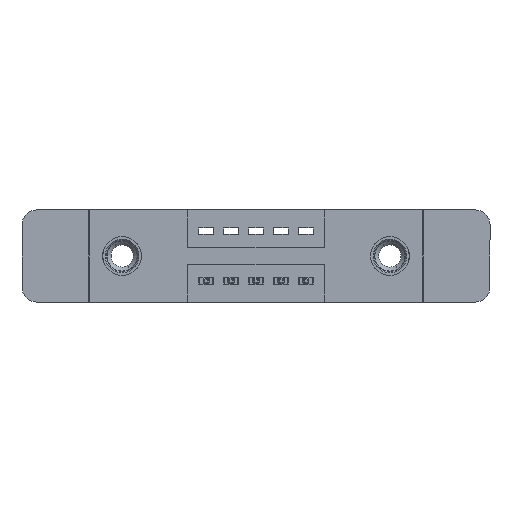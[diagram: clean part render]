
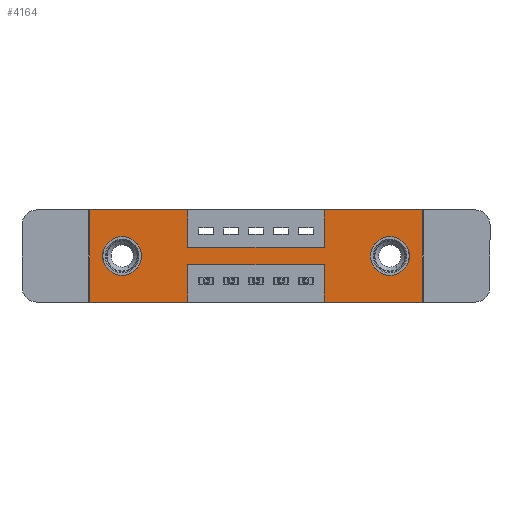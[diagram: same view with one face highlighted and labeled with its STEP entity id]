
A CAD part, front view. The second image highlights one B-rep face of the part: STEP entity #4164.
In plain terms, the highlighted planar face has unit normal (0, -1, 0).
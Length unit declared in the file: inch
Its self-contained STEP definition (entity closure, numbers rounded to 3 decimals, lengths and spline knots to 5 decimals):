
#6 = VERTEX_POINT ( 'NONE', #2094 ) ;
#29 = LINE ( 'NONE', #2157, #3273 ) ;
#274 = EDGE_CURVE ( 'NONE', #6, #1715, #13702, .T. ) ;
#419 = LINE ( 'NONE', #6791, #4056 ) ;
#558 = DIRECTION ( 'NONE',  ( 0., 1., 0. ) ) ;
#1083 = ORIENTED_EDGE ( 'NONE', *, *, #10503, .F. ) ;
#1198 = EDGE_CURVE ( 'NONE', #1715, #6, #1254, .T. ) ;
#1203 = DIRECTION ( 'NONE',  ( 0., 0., -1. ) ) ;
#1254 = CIRCLE ( 'NONE', #9157, 0.078 ) ;
#1286 = ORIENTED_EDGE ( 'NONE', *, *, #3665, .F. ) ;
#1483 = EDGE_CURVE ( 'NONE', #9613, #10770, #11047, .T. ) ;
#1488 = AXIS2_PLACEMENT_3D ( 'NONE', #5794, #558, #7996 ) ;
#1510 = CARTESIAN_POINT ( 'NONE',  ( 0.3925, 0., -0.22 ) ) ;
#1560 = DIRECTION ( 'NONE',  ( 0., 0., -1. ) ) ;
#1562 = CARTESIAN_POINT ( 'NONE',  ( 0.13, 0., -0.107 ) ) ;
#1658 = CARTESIAN_POINT ( 'NONE',  ( 1.205, 0., -0.185 ) ) ;
#1715 = VERTEX_POINT ( 'NONE', #10465 ) ;
#1726 = LINE ( 'NONE', #11574, #4717 ) ;
#2094 = CARTESIAN_POINT ( 'NONE',  ( 1.205, 0., -0.107 ) ) ;
#2152 = LINE ( 'NONE', #8588, #6962 ) ;
#2157 = CARTESIAN_POINT ( 'NONE',  ( 0., 0., 0. ) ) ;
#2164 = ORIENTED_EDGE ( 'NONE', *, *, #6714, .T. ) ;
#2432 = LINE ( 'NONE', #5740, #12918 ) ;
#2612 = FACE_OUTER_BOUND ( 'NONE', #13594, .T. ) ;
#2771 = LINE ( 'NONE', #5170, #13101 ) ;
#2775 = ORIENTED_EDGE ( 'NONE', *, *, #3878, .F. ) ;
#2916 = EDGE_LOOP ( 'NONE', ( #2164, #5886 ) ) ;
#3038 = DIRECTION ( 'NONE',  ( 1., 0., 0. ) ) ;
#3239 = CARTESIAN_POINT ( 'NONE',  ( 0.13, 0., -0.263 ) ) ;
#3273 = VECTOR ( 'NONE', #6478, 39.37008 ) ;
#3569 = DIRECTION ( 'NONE',  ( -1., 0., 0. ) ) ;
#3665 = EDGE_CURVE ( 'NONE', #7638, #11345, #2152, .T. ) ;
#3668 = ORIENTED_EDGE ( 'NONE', *, *, #10393, .F. ) ;
#3686 = VERTEX_POINT ( 'NONE', #11650 ) ;
#3878 = EDGE_CURVE ( 'NONE', #9111, #9617, #13063, .T. ) ;
#3971 = DIRECTION ( 'NONE',  ( 1., 0., 0. ) ) ;
#4056 = VECTOR ( 'NONE', #6647, 39.37008 ) ;
#4164 = ADVANCED_FACE ( 'NONE', ( #9041, #13456, #2612 ), #5711, .T. ) ;
#4335 = ORIENTED_EDGE ( 'NONE', *, *, #1483, .F. ) ;
#4374 = ORIENTED_EDGE ( 'NONE', *, *, #12485, .F. ) ;
#4717 = VECTOR ( 'NONE', #10267, 39.37008 ) ;
#4948 = DIRECTION ( 'NONE',  ( -1., 0., 0. ) ) ;
#4963 = DIRECTION ( 'NONE',  ( 0., 0., 1. ) ) ;
#5170 = CARTESIAN_POINT ( 'NONE',  ( 0., 0., 0. ) ) ;
#5299 = CARTESIAN_POINT ( 'NONE',  ( 0., 0., 0. ) ) ;
#5468 = EDGE_CURVE ( 'NONE', #9166, #9613, #29, .T. ) ;
#5510 = CARTESIAN_POINT ( 'NONE',  ( 0.9425, 0., -0.15 ) ) ;
#5711 = PLANE ( 'NONE',  #8988 ) ;
#5721 = LINE ( 'NONE', #10535, #12345 ) ;
#5740 = CARTESIAN_POINT ( 'NONE',  ( 0.9425, 0., 0. ) ) ;
#5794 = CARTESIAN_POINT ( 'NONE',  ( 0.13, 0., -0.185 ) ) ;
#5832 = VERTEX_POINT ( 'NONE', #3239 ) ;
#5886 = ORIENTED_EDGE ( 'NONE', *, *, #10207, .T. ) ;
#5976 = DIRECTION ( 'NONE',  ( 0., 1., 0. ) ) ;
#6117 = DIRECTION ( 'NONE',  ( 0., 0., -1. ) ) ;
#6469 = DIRECTION ( 'NONE',  ( 0., 0., -1. ) ) ;
#6478 = DIRECTION ( 'NONE',  ( 1., 0., 0. ) ) ;
#6503 = LINE ( 'NONE', #11026, #9245 ) ;
#6577 = DIRECTION ( 'NONE',  ( 0., 0., -1. ) ) ;
#6647 = DIRECTION ( 'NONE',  ( -1., 0., 0. ) ) ;
#6714 = EDGE_CURVE ( 'NONE', #11472, #5832, #11659, .T. ) ;
#6791 = CARTESIAN_POINT ( 'NONE',  ( 0., 0., -0.37 ) ) ;
#6852 = EDGE_CURVE ( 'NONE', #10770, #11330, #5721, .T. ) ;
#6912 = AXIS2_PLACEMENT_3D ( 'NONE', #1658, #9142, #6117 ) ;
#6962 = VECTOR ( 'NONE', #6469, 39.37008 ) ;
#7040 = VERTEX_POINT ( 'NONE', #11822 ) ;
#7179 = ORIENTED_EDGE ( 'NONE', *, *, #1198, .T. ) ;
#7638 = VERTEX_POINT ( 'NONE', #9150 ) ;
#7996 = DIRECTION ( 'NONE',  ( 0., 0., 1. ) ) ;
#8115 = VECTOR ( 'NONE', #13775, 39.37008 ) ;
#8167 = EDGE_LOOP ( 'NONE', ( #8419, #7179 ) ) ;
#8419 = ORIENTED_EDGE ( 'NONE', *, *, #274, .T. ) ;
#8588 = CARTESIAN_POINT ( 'NONE',  ( 1.335, 0., 0. ) ) ;
#8703 = ORIENTED_EDGE ( 'NONE', *, *, #10226, .F. ) ;
#8909 = EDGE_CURVE ( 'NONE', #11330, #7040, #2432, .T. ) ;
#8923 = CARTESIAN_POINT ( 'NONE',  ( 0.3925, 0., -0.22 ) ) ;
#8988 = AXIS2_PLACEMENT_3D ( 'NONE', #12177, #10020, #1560 ) ;
#9041 = FACE_BOUND ( 'NONE', #8167, .T. ) ;
#9111 = VERTEX_POINT ( 'NONE', #13028 ) ;
#9142 = DIRECTION ( 'NONE',  ( 0., 1., 0. ) ) ;
#9150 = CARTESIAN_POINT ( 'NONE',  ( 1.335, 0., 0. ) ) ;
#9154 = CARTESIAN_POINT ( 'NONE',  ( 1.205, 0., -0.185 ) ) ;
#9157 = AXIS2_PLACEMENT_3D ( 'NONE', #9154, #5976, #9233 ) ;
#9166 = VERTEX_POINT ( 'NONE', #5299 ) ;
#9233 = DIRECTION ( 'NONE',  ( 0., 0., -1. ) ) ;
#9240 = ORIENTED_EDGE ( 'NONE', *, *, #6852, .F. ) ;
#9241 = AXIS2_PLACEMENT_3D ( 'NONE', #12621, #12690, #4963 ) ;
#9245 = VECTOR ( 'NONE', #6577, 39.37008 ) ;
#9353 = VERTEX_POINT ( 'NONE', #12248 ) ;
#9461 = VECTOR ( 'NONE', #4948, 39.37008 ) ;
#9613 = VERTEX_POINT ( 'NONE', #10986 ) ;
#9617 = VERTEX_POINT ( 'NONE', #1510 ) ;
#9988 = DIRECTION ( 'NONE',  ( 0., 0., 1. ) ) ;
#10020 = DIRECTION ( 'NONE',  ( 0., -1., 0. ) ) ;
#10155 = CARTESIAN_POINT ( 'NONE',  ( 0.3925, 0., -0.37 ) ) ;
#10207 = EDGE_CURVE ( 'NONE', #5832, #11472, #13786, .T. ) ;
#10226 = EDGE_CURVE ( 'NONE', #7040, #7638, #2771, .T. ) ;
#10267 = DIRECTION ( 'NONE',  ( 0., 0., 1. ) ) ;
#10393 = EDGE_CURVE ( 'NONE', #11863, #9353, #419, .T. ) ;
#10465 = CARTESIAN_POINT ( 'NONE',  ( 1.205, 0., -0.263 ) ) ;
#10503 = EDGE_CURVE ( 'NONE', #11345, #3686, #13736, .T. ) ;
#10510 = ORIENTED_EDGE ( 'NONE', *, *, #13298, .F. ) ;
#10535 = CARTESIAN_POINT ( 'NONE',  ( 0.3925, 0., -0.15 ) ) ;
#10744 = VECTOR ( 'NONE', #1203, 39.37008 ) ;
#10770 = VERTEX_POINT ( 'NONE', #12514 ) ;
#10986 = CARTESIAN_POINT ( 'NONE',  ( 0.3925, 0., 0. ) ) ;
#11026 = CARTESIAN_POINT ( 'NONE',  ( 0.3925, 0., -0.37 ) ) ;
#11047 = LINE ( 'NONE', #12265, #10744 ) ;
#11113 = ORIENTED_EDGE ( 'NONE', *, *, #12414, .F. ) ;
#11330 = VERTEX_POINT ( 'NONE', #5510 ) ;
#11345 = VERTEX_POINT ( 'NONE', #12900 ) ;
#11357 = LINE ( 'NONE', #12640, #8115 ) ;
#11434 = ORIENTED_EDGE ( 'NONE', *, *, #8909, .F. ) ;
#11472 = VERTEX_POINT ( 'NONE', #1562 ) ;
#11574 = CARTESIAN_POINT ( 'NONE',  ( 0., 0., 0. ) ) ;
#11605 = CARTESIAN_POINT ( 'NONE',  ( 0., 0., -0.37 ) ) ;
#11650 = CARTESIAN_POINT ( 'NONE',  ( 0.9425, 0., -0.37 ) ) ;
#11659 = CIRCLE ( 'NONE', #1488, 0.078 ) ;
#11822 = CARTESIAN_POINT ( 'NONE',  ( 0.9425, 0., 0. ) ) ;
#11863 = VERTEX_POINT ( 'NONE', #10155 ) ;
#12177 = CARTESIAN_POINT ( 'NONE',  ( 0., 0., -0.37 ) ) ;
#12248 = CARTESIAN_POINT ( 'NONE',  ( 0., 0., -0.37 ) ) ;
#12265 = CARTESIAN_POINT ( 'NONE',  ( 0.3925, 0., 0. ) ) ;
#12345 = VECTOR ( 'NONE', #3038, 39.37008 ) ;
#12383 = ORIENTED_EDGE ( 'NONE', *, *, #5468, .F. ) ;
#12411 = VECTOR ( 'NONE', #3569, 39.37008 ) ;
#12414 = EDGE_CURVE ( 'NONE', #9353, #9166, #1726, .T. ) ;
#12485 = EDGE_CURVE ( 'NONE', #3686, #9111, #11357, .T. ) ;
#12514 = CARTESIAN_POINT ( 'NONE',  ( 0.3925, 0., -0.15 ) ) ;
#12621 = CARTESIAN_POINT ( 'NONE',  ( 0.13, 0., -0.185 ) ) ;
#12640 = CARTESIAN_POINT ( 'NONE',  ( 0.9425, 0., -0.37 ) ) ;
#12690 = DIRECTION ( 'NONE',  ( 0., 1., 0. ) ) ;
#12900 = CARTESIAN_POINT ( 'NONE',  ( 1.335, 0., -0.37 ) ) ;
#12918 = VECTOR ( 'NONE', #9988, 39.37008 ) ;
#13028 = CARTESIAN_POINT ( 'NONE',  ( 0.9425, 0., -0.22 ) ) ;
#13063 = LINE ( 'NONE', #8923, #12411 ) ;
#13101 = VECTOR ( 'NONE', #3971, 39.37008 ) ;
#13298 = EDGE_CURVE ( 'NONE', #9617, #11863, #6503, .T. ) ;
#13456 = FACE_BOUND ( 'NONE', #2916, .T. ) ;
#13594 = EDGE_LOOP ( 'NONE', ( #10510, #2775, #4374, #1083, #1286, #8703, #11434, #9240, #4335, #12383, #11113, #3668 ) ) ;
#13702 = CIRCLE ( 'NONE', #6912, 0.078 ) ;
#13736 = LINE ( 'NONE', #11605, #9461 ) ;
#13775 = DIRECTION ( 'NONE',  ( 0., 0., 1. ) ) ;
#13786 = CIRCLE ( 'NONE', #9241, 0.078 ) ;
